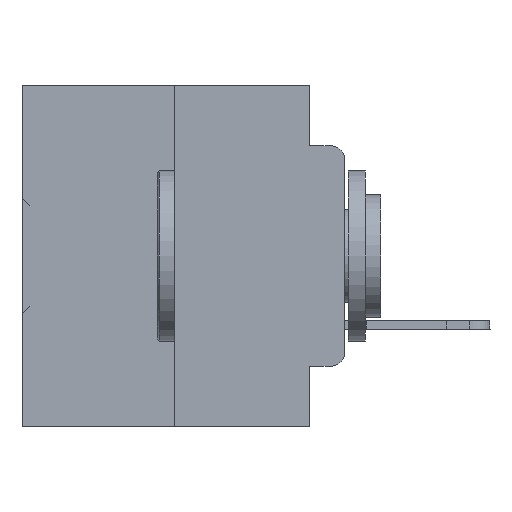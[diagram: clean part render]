
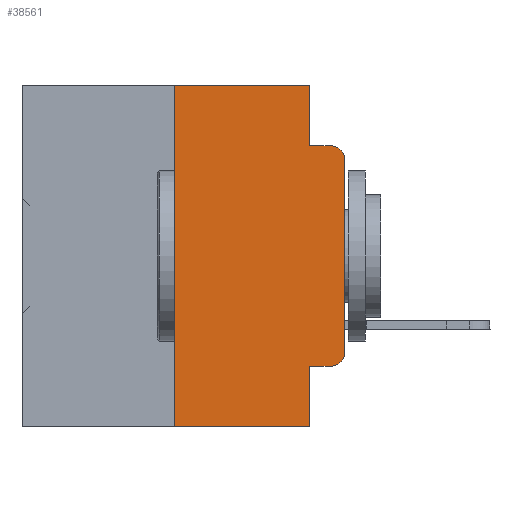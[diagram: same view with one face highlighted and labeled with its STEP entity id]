
A CAD part, left-side view. The second image highlights one B-rep face of the part: STEP entity #38561.
In plain terms, the highlighted planar face has unit normal (-1, 0, 0).
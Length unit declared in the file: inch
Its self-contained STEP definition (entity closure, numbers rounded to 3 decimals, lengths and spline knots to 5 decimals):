
#1360 = VECTOR ( 'NONE', #13301, 39.37008 ) ;
#1477 = LINE ( 'NONE', #15959, #30379 ) ;
#2356 = EDGE_CURVE ( 'NONE', #5507, #12604, #24754, .T. ) ;
#2505 = EDGE_CURVE ( 'NONE', #31823, #36805, #1477, .T. ) ;
#2528 = EDGE_CURVE ( 'NONE', #23720, #19582, #30985, .T. ) ;
#2932 = CARTESIAN_POINT ( 'NONE',  ( 0., 0.051, -0.0885 ) ) ;
#2977 = DIRECTION ( 'NONE',  ( 0., 0., 1. ) ) ;
#3339 = DIRECTION ( 'NONE',  ( 0., -1., 0. ) ) ;
#3821 = ORIENTED_EDGE ( 'NONE', *, *, #29224, .F. ) ;
#4273 = CARTESIAN_POINT ( 'NONE',  ( 0., 0.25, 0. ) ) ;
#4364 = CARTESIAN_POINT ( 'NONE',  ( 0., 0.473, -0.5 ) ) ;
#4563 = AXIS2_PLACEMENT_3D ( 'NONE', #6286, #15637, #18181 ) ;
#4796 = AXIS2_PLACEMENT_3D ( 'NONE', #18124, #26903, #12834 ) ;
#5171 = CARTESIAN_POINT ( 'NONE',  ( 0., 0.02, -0.4115 ) ) ;
#5369 = EDGE_CURVE ( 'NONE', #11370, #5507, #22344, .T. ) ;
#5507 = VERTEX_POINT ( 'NONE', #5171 ) ;
#6286 = CARTESIAN_POINT ( 'NONE',  ( 0., 0.473, 0. ) ) ;
#6557 = ORIENTED_EDGE ( 'NONE', *, *, #23252, .T. ) ;
#8525 = CARTESIAN_POINT ( 'NONE',  ( 0., 0.051, -0.0885 ) ) ;
#8932 = VECTOR ( 'NONE', #13196, 39.37008 ) ;
#9138 = ORIENTED_EDGE ( 'NONE', *, *, #11010, .T. ) ;
#9623 = VERTEX_POINT ( 'NONE', #15953 ) ;
#9959 = PLANE ( 'NONE',  #4563 ) ;
#10518 = ORIENTED_EDGE ( 'NONE', *, *, #34298, .T. ) ;
#11010 = EDGE_CURVE ( 'NONE', #33967, #9623, #21720, .T. ) ;
#11370 = VERTEX_POINT ( 'NONE', #14908 ) ;
#11959 = CARTESIAN_POINT ( 'NONE',  ( 0., 0., 0. ) ) ;
#12289 = VECTOR ( 'NONE', #33885, 39.37008 ) ;
#12604 = VERTEX_POINT ( 'NONE', #34130 ) ;
#12834 = DIRECTION ( 'NONE',  ( 0., 0., -1. ) ) ;
#13196 = DIRECTION ( 'NONE',  ( 0., -1., 0. ) ) ;
#13301 = DIRECTION ( 'NONE',  ( 0., 0., -1. ) ) ;
#14908 = CARTESIAN_POINT ( 'NONE',  ( 0., 0.051, -0.4115 ) ) ;
#15637 = DIRECTION ( 'NONE',  ( 1., 0., 0. ) ) ;
#15716 = VECTOR ( 'NONE', #3339, 39.37008 ) ;
#15953 = CARTESIAN_POINT ( 'NONE',  ( 0., 0.02, -0.0885 ) ) ;
#15959 = CARTESIAN_POINT ( 'NONE',  ( 0., 0.25, 0. ) ) ;
#15974 = EDGE_CURVE ( 'NONE', #11370, #32606, #16421, .T. ) ;
#16180 = CARTESIAN_POINT ( 'NONE',  ( 0., 0.051, 0. ) ) ;
#16276 = DIRECTION ( 'NONE',  ( 0., -1., 0. ) ) ;
#16421 = LINE ( 'NONE', #27749, #1360 ) ;
#16809 = ORIENTED_EDGE ( 'NONE', *, *, #5369, .T. ) ;
#18015 = VECTOR ( 'NONE', #35642, 39.37008 ) ;
#18124 = CARTESIAN_POINT ( 'NONE',  ( 0., 0.02, -0.3915 ) ) ;
#18181 = DIRECTION ( 'NONE',  ( 0., 0., -1. ) ) ;
#18255 = ORIENTED_EDGE ( 'NONE', *, *, #2356, .T. ) ;
#19124 = VECTOR ( 'NONE', #2977, 39.37008 ) ;
#19582 = VERTEX_POINT ( 'NONE', #2932 ) ;
#20882 = LINE ( 'NONE', #30264, #15716 ) ;
#21720 = CIRCLE ( 'NONE', #23576, 0.02 ) ;
#21995 = CARTESIAN_POINT ( 'NONE',  ( 0., 0.051, 0. ) ) ;
#22344 = LINE ( 'NONE', #36802, #8932 ) ;
#23252 = EDGE_CURVE ( 'NONE', #12604, #33967, #29706, .T. ) ;
#23576 = AXIS2_PLACEMENT_3D ( 'NONE', #36779, #34017, #33652 ) ;
#23720 = VERTEX_POINT ( 'NONE', #16180 ) ;
#24754 = CIRCLE ( 'NONE', #4796, 0.02 ) ;
#24864 = LINE ( 'NONE', #4364, #24992 ) ;
#24992 = VECTOR ( 'NONE', #16276, 39.37008 ) ;
#25307 = DIRECTION ( 'NONE',  ( 0., 0., 1. ) ) ;
#26808 = EDGE_LOOP ( 'NONE', ( #6557, #9138, #29367, #31252, #3821, #34870, #10518, #29127, #16809, #18255 ) ) ;
#26903 = DIRECTION ( 'NONE',  ( -1., 0., 0. ) ) ;
#27543 = CARTESIAN_POINT ( 'NONE',  ( 0., 0., -0.1085 ) ) ;
#27749 = CARTESIAN_POINT ( 'NONE',  ( 0., 0.051, 0. ) ) ;
#28818 = CARTESIAN_POINT ( 'NONE',  ( 0., 0.25, -0.5 ) ) ;
#28901 = CARTESIAN_POINT ( 'NONE',  ( 0., 0.051, -0.5 ) ) ;
#29127 = ORIENTED_EDGE ( 'NONE', *, *, #15974, .F. ) ;
#29224 = EDGE_CURVE ( 'NONE', #36805, #23720, #20882, .T. ) ;
#29367 = ORIENTED_EDGE ( 'NONE', *, *, #31976, .F. ) ;
#29706 = LINE ( 'NONE', #11959, #19124 ) ;
#30264 = CARTESIAN_POINT ( 'NONE',  ( 0., 0.473, 0. ) ) ;
#30379 = VECTOR ( 'NONE', #25307, 39.37008 ) ;
#30985 = LINE ( 'NONE', #21995, #12289 ) ;
#31252 = ORIENTED_EDGE ( 'NONE', *, *, #2528, .F. ) ;
#31823 = VERTEX_POINT ( 'NONE', #28818 ) ;
#31976 = EDGE_CURVE ( 'NONE', #19582, #9623, #38585, .T. ) ;
#32606 = VERTEX_POINT ( 'NONE', #28901 ) ;
#33652 = DIRECTION ( 'NONE',  ( 0., 0., -1. ) ) ;
#33885 = DIRECTION ( 'NONE',  ( 0., 0., -1. ) ) ;
#33967 = VERTEX_POINT ( 'NONE', #27543 ) ;
#34017 = DIRECTION ( 'NONE',  ( -1., 0., 0. ) ) ;
#34130 = CARTESIAN_POINT ( 'NONE',  ( 0., 0., -0.3915 ) ) ;
#34298 = EDGE_CURVE ( 'NONE', #31823, #32606, #24864, .T. ) ;
#34870 = ORIENTED_EDGE ( 'NONE', *, *, #2505, .F. ) ;
#35642 = DIRECTION ( 'NONE',  ( 0., -1., 0. ) ) ;
#36329 = FACE_OUTER_BOUND ( 'NONE', #26808, .T. ) ;
#36779 = CARTESIAN_POINT ( 'NONE',  ( 0., 0.02, -0.1085 ) ) ;
#36802 = CARTESIAN_POINT ( 'NONE',  ( 0., 0.051, -0.4115 ) ) ;
#36805 = VERTEX_POINT ( 'NONE', #4273 ) ;
#38561 = ADVANCED_FACE ( 'NONE', ( #36329 ), #9959, .F. ) ;
#38585 = LINE ( 'NONE', #8525, #18015 ) ;
